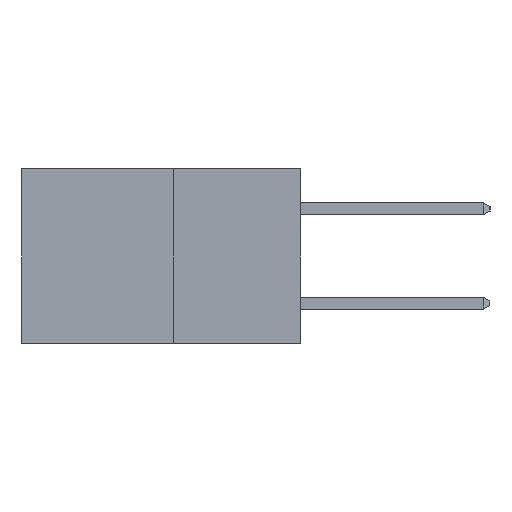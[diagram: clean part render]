
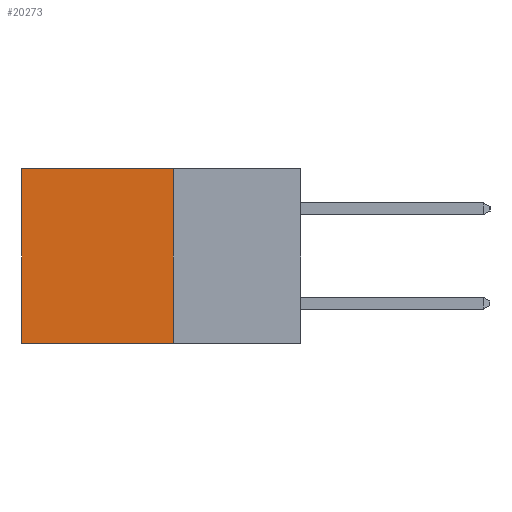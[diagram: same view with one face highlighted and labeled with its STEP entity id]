
A CAD part, left-side view. The second image highlights one B-rep face of the part: STEP entity #20273.
In plain terms, the highlighted planar face has unit normal (-1, 0, 0).
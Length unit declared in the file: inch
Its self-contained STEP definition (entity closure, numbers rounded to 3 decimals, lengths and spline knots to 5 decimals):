
#78 = VECTOR ( 'NONE', #24785, 39.37008 ) ;
#1319 = LINE ( 'NONE', #12866, #18149 ) ;
#1492 = VERTEX_POINT ( 'NONE', #26896 ) ;
#3774 = ORIENTED_EDGE ( 'NONE', *, *, #26260, .F. ) ;
#5423 = LINE ( 'NONE', #8763, #78 ) ;
#6516 = VECTOR ( 'NONE', #7555, 39.37008 ) ;
#6981 = CARTESIAN_POINT ( 'NONE',  ( 0.277, 0.27, 0. ) ) ;
#7555 = DIRECTION ( 'NONE',  ( 0., 0., -1. ) ) ;
#7684 = ORIENTED_EDGE ( 'NONE', *, *, #9509, .T. ) ;
#7840 = EDGE_LOOP ( 'NONE', ( #7684, #26671, #3774, #29568 ) ) ;
#8763 = CARTESIAN_POINT ( 'NONE',  ( 0.277, 0.27, -0.37 ) ) ;
#8980 = CARTESIAN_POINT ( 'NONE',  ( 0.277, 0.27, -0.37 ) ) ;
#9509 = EDGE_CURVE ( 'NONE', #12516, #17097, #18712, .T. ) ;
#11282 = DIRECTION ( 'NONE',  ( 0., 0., -1. ) ) ;
#11447 = CARTESIAN_POINT ( 'NONE',  ( 0.277, 0.59, 0. ) ) ;
#12516 = VERTEX_POINT ( 'NONE', #11447 ) ;
#12866 = CARTESIAN_POINT ( 'NONE',  ( 0.277, 0.27, 0. ) ) ;
#15287 = EDGE_CURVE ( 'NONE', #1492, #17097, #25790, .T. ) ;
#15373 = CARTESIAN_POINT ( 'NONE',  ( 0.277, 0.27, -0.37 ) ) ;
#17097 = VERTEX_POINT ( 'NONE', #18190 ) ;
#17870 = DIRECTION ( 'NONE',  ( 0., 1., 0. ) ) ;
#18149 = VECTOR ( 'NONE', #28868, 39.37008 ) ;
#18190 = CARTESIAN_POINT ( 'NONE',  ( 0.277, 0.59, -0.37 ) ) ;
#18712 = LINE ( 'NONE', #23578, #6516 ) ;
#19697 = VECTOR ( 'NONE', #17870, 39.37008 ) ;
#20273 = ADVANCED_FACE ( 'NONE', ( #29411 ), #22662, .F. ) ;
#21632 = VERTEX_POINT ( 'NONE', #6981 ) ;
#22662 = PLANE ( 'NONE',  #23537 ) ;
#22672 = EDGE_CURVE ( 'NONE', #21632, #12516, #1319, .T. ) ;
#23537 = AXIS2_PLACEMENT_3D ( 'NONE', #8980, #25002, #11282 ) ;
#23578 = CARTESIAN_POINT ( 'NONE',  ( 0.277, 0.59, -0.37 ) ) ;
#24785 = DIRECTION ( 'NONE',  ( 0., 0., -1. ) ) ;
#25002 = DIRECTION ( 'NONE',  ( 1., 0., 0. ) ) ;
#25790 = LINE ( 'NONE', #15373, #19697 ) ;
#26260 = EDGE_CURVE ( 'NONE', #21632, #1492, #5423, .T. ) ;
#26671 = ORIENTED_EDGE ( 'NONE', *, *, #15287, .F. ) ;
#26896 = CARTESIAN_POINT ( 'NONE',  ( 0.277, 0.27, -0.37 ) ) ;
#28868 = DIRECTION ( 'NONE',  ( 0., 1., 0. ) ) ;
#29411 = FACE_OUTER_BOUND ( 'NONE', #7840, .T. ) ;
#29568 = ORIENTED_EDGE ( 'NONE', *, *, #22672, .T. ) ;
